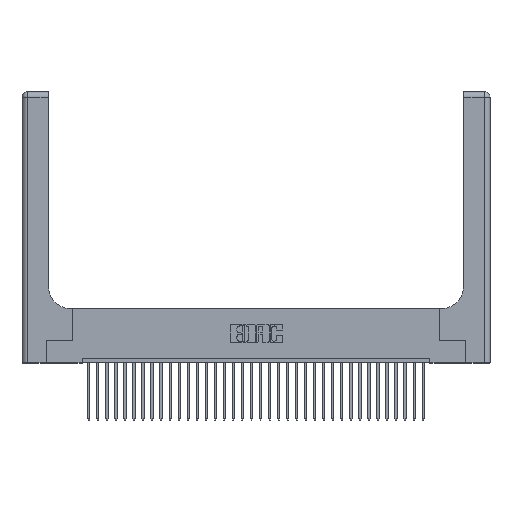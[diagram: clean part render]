
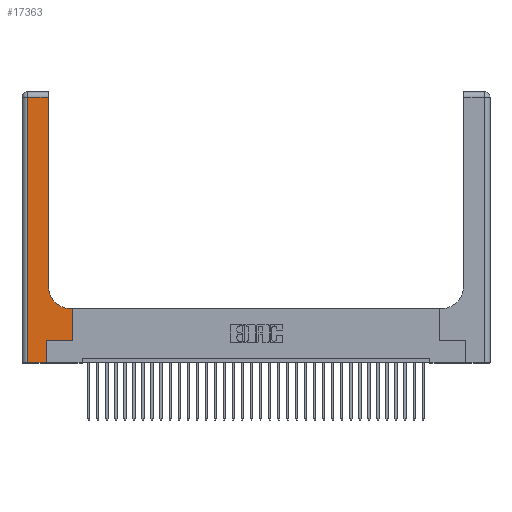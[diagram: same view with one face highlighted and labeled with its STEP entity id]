
A CAD part, top view. The second image highlights one B-rep face of the part: STEP entity #17363.
In plain terms, the highlighted planar face has unit normal (0, 0, 1).
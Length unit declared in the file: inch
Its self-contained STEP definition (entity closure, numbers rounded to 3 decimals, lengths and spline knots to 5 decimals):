
#436 = CARTESIAN_POINT ( 'NONE',  ( 0.5415, 0.85, 0.37 ) ) ;
#1420 = CARTESIAN_POINT ( 'NONE',  ( 0.2915, 2.94, 0.37 ) ) ;
#1857 = DIRECTION ( 'NONE',  ( -1., 0., 0. ) ) ;
#2015 = VERTEX_POINT ( 'NONE', #14633 ) ;
#2258 = CARTESIAN_POINT ( 'NONE',  ( 0.2915, 3., 0.37 ) ) ;
#2304 = VERTEX_POINT ( 'NONE', #22113 ) ;
#2765 = DIRECTION ( 'NONE',  ( -1., 0., 0. ) ) ;
#2938 = CARTESIAN_POINT ( 'NONE',  ( 0., 0., 0.37 ) ) ;
#3113 = DIRECTION ( 'NONE',  ( 0., 0., -1. ) ) ;
#3322 = CARTESIAN_POINT ( 'NONE',  ( 0.269, 0.25, 0.37 ) ) ;
#3673 = VERTEX_POINT ( 'NONE', #9844 ) ;
#3889 = DIRECTION ( 'NONE',  ( 0., 1., 0. ) ) ;
#4011 = DIRECTION ( 'NONE',  ( 1., 0., 0. ) ) ;
#4129 = DIRECTION ( 'NONE',  ( 1., 0., 0. ) ) ;
#4264 = CIRCLE ( 'NONE', #26612, 0.25 ) ;
#4973 = CARTESIAN_POINT ( 'NONE',  ( 0.06, 2.94, 0.37 ) ) ;
#5600 = EDGE_CURVE ( 'NONE', #15369, #2304, #24630, .T. ) ;
#6121 = EDGE_LOOP ( 'NONE', ( #29942, #25241, #7331, #18782, #22999, #17334, #29305, #21581, #31789 ) ) ;
#6249 = PLANE ( 'NONE',  #21875 ) ;
#6693 = CARTESIAN_POINT ( 'NONE',  ( 0.269, 0.25, 0.37 ) ) ;
#6764 = VECTOR ( 'NONE', #4011, 39.37008 ) ;
#7331 = ORIENTED_EDGE ( 'NONE', *, *, #14834, .T. ) ;
#7486 = VECTOR ( 'NONE', #3889, 39.37008 ) ;
#8070 = EDGE_CURVE ( 'NONE', #3673, #15369, #10684, .T. ) ;
#8711 = CARTESIAN_POINT ( 'NONE',  ( 0., 3., 0.37 ) ) ;
#9569 = CARTESIAN_POINT ( 'NONE',  ( 0.2915, 0.85, 0.37 ) ) ;
#9844 = CARTESIAN_POINT ( 'NONE',  ( 0.5585, 0.25, 0.37 ) ) ;
#10684 = LINE ( 'NONE', #33955, #22722 ) ;
#11594 = DIRECTION ( 'NONE',  ( 0., 0., -1. ) ) ;
#11614 = FACE_OUTER_BOUND ( 'NONE', #6121, .T. ) ;
#12444 = EDGE_CURVE ( 'NONE', #30367, #16983, #14519, .T. ) ;
#12452 = EDGE_CURVE ( 'NONE', #16983, #3673, #27360, .T. ) ;
#13039 = LINE ( 'NONE', #26581, #26689 ) ;
#14163 = DIRECTION ( 'NONE',  ( -1., 0., 0. ) ) ;
#14336 = LINE ( 'NONE', #17070, #17670 ) ;
#14519 = LINE ( 'NONE', #27685, #7486 ) ;
#14633 = CARTESIAN_POINT ( 'NONE',  ( 0.06, 0., 0.37 ) ) ;
#14834 = EDGE_CURVE ( 'NONE', #25216, #2015, #14336, .T. ) ;
#15369 = VERTEX_POINT ( 'NONE', #16619 ) ;
#15960 = VECTOR ( 'NONE', #18837, 39.37008 ) ;
#16151 = VERTEX_POINT ( 'NONE', #1420 ) ;
#16219 = EDGE_CURVE ( 'NONE', #2015, #30367, #28338, .T. ) ;
#16619 = CARTESIAN_POINT ( 'NONE',  ( 0.5585, 0.6, 0.37 ) ) ;
#16983 = VERTEX_POINT ( 'NONE', #3322 ) ;
#17070 = CARTESIAN_POINT ( 'NONE',  ( 0.06, 3., 0.37 ) ) ;
#17334 = ORIENTED_EDGE ( 'NONE', *, *, #12452, .T. ) ;
#17363 = ADVANCED_FACE ( 'NONE', ( #11614 ), #6249, .F. ) ;
#17670 = VECTOR ( 'NONE', #31190, 39.37008 ) ;
#18782 = ORIENTED_EDGE ( 'NONE', *, *, #16219, .T. ) ;
#18837 = DIRECTION ( 'NONE',  ( 0., 1., 0. ) ) ;
#21001 = DIRECTION ( 'NONE',  ( 0., 1., 0. ) ) ;
#21581 = ORIENTED_EDGE ( 'NONE', *, *, #5600, .T. ) ;
#21755 = EDGE_CURVE ( 'NONE', #25880, #16151, #23842, .T. ) ;
#21875 = AXIS2_PLACEMENT_3D ( 'NONE', #8711, #11594, #14163 ) ;
#22113 = CARTESIAN_POINT ( 'NONE',  ( 0.5415, 0.6, 0.37 ) ) ;
#22722 = VECTOR ( 'NONE', #21001, 39.37008 ) ;
#22999 = ORIENTED_EDGE ( 'NONE', *, *, #12444, .T. ) ;
#23609 = CARTESIAN_POINT ( 'NONE',  ( 0.269, 0., 0.37 ) ) ;
#23842 = LINE ( 'NONE', #2258, #15960 ) ;
#24466 = VECTOR ( 'NONE', #4129, 39.37008 ) ;
#24630 = LINE ( 'NONE', #25558, #25050 ) ;
#25050 = VECTOR ( 'NONE', #1857, 39.37008 ) ;
#25216 = VERTEX_POINT ( 'NONE', #4973 ) ;
#25241 = ORIENTED_EDGE ( 'NONE', *, *, #30524, .T. ) ;
#25558 = CARTESIAN_POINT ( 'NONE',  ( 0.2915, 0.6, 0.37 ) ) ;
#25880 = VERTEX_POINT ( 'NONE', #9569 ) ;
#26581 = CARTESIAN_POINT ( 'NONE',  ( 0., 2.94, 0.37 ) ) ;
#26612 = AXIS2_PLACEMENT_3D ( 'NONE', #436, #3113, #29335 ) ;
#26689 = VECTOR ( 'NONE', #2765, 39.37008 ) ;
#27360 = LINE ( 'NONE', #6693, #24466 ) ;
#27685 = CARTESIAN_POINT ( 'NONE',  ( 0.269, 0., 0.37 ) ) ;
#28338 = LINE ( 'NONE', #2938, #6764 ) ;
#29305 = ORIENTED_EDGE ( 'NONE', *, *, #8070, .T. ) ;
#29335 = DIRECTION ( 'NONE',  ( 1., 0., 0. ) ) ;
#29942 = ORIENTED_EDGE ( 'NONE', *, *, #21755, .T. ) ;
#30367 = VERTEX_POINT ( 'NONE', #23609 ) ;
#30524 = EDGE_CURVE ( 'NONE', #16151, #25216, #13039, .T. ) ;
#30539 = EDGE_CURVE ( 'NONE', #2304, #25880, #4264, .T. ) ;
#31190 = DIRECTION ( 'NONE',  ( 0., -1., 0. ) ) ;
#31789 = ORIENTED_EDGE ( 'NONE', *, *, #30539, .T. ) ;
#33955 = CARTESIAN_POINT ( 'NONE',  ( 0.5585, 0.25, 0.37 ) ) ;
